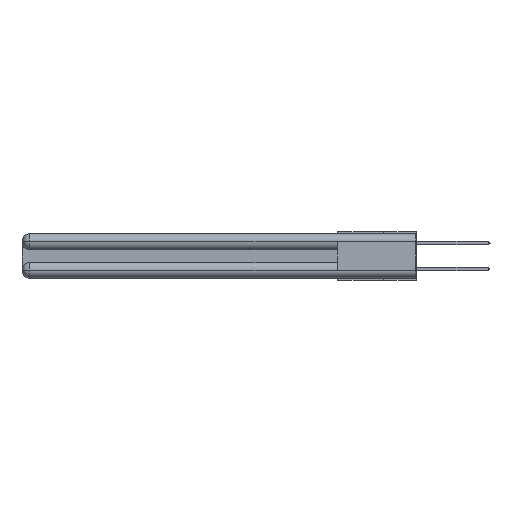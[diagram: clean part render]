
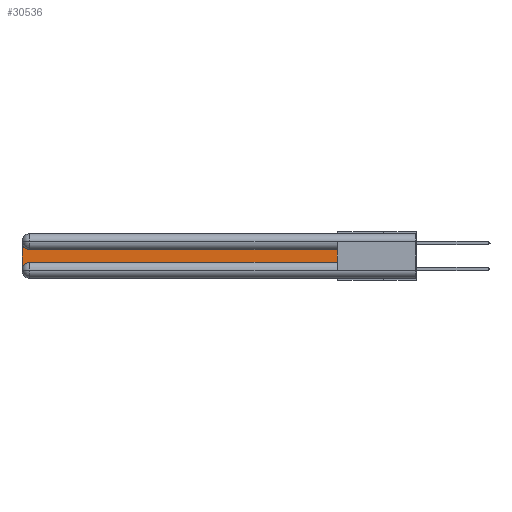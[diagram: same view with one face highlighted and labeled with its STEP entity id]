
A CAD part, left-side view. The second image highlights one B-rep face of the part: STEP entity #30536.
In plain terms, the highlighted planar face has unit normal (-1, 0, 0).
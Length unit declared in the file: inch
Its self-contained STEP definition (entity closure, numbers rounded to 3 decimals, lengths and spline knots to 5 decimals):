
#1309 = LINE ( 'NONE', #4899, #30831 ) ;
#1472 = DIRECTION ( 'NONE',  ( 0., 0., -1. ) ) ;
#1687 = EDGE_CURVE ( 'NONE', #29942, #4841, #17543, .T. ) ;
#2411 = CARTESIAN_POINT ( 'NONE',  ( 0.075, 2.94, -0.2175 ) ) ;
#2611 = CARTESIAN_POINT ( 'NONE',  ( 0.075, 0.6, -0.2175 ) ) ;
#3957 = CIRCLE ( 'NONE', #18396, 0.06 ) ;
#4057 = PLANE ( 'NONE',  #16762 ) ;
#4304 = DIRECTION ( 'NONE',  ( 0., 0., -1. ) ) ;
#4841 = VERTEX_POINT ( 'NONE', #32717 ) ;
#4899 = CARTESIAN_POINT ( 'NONE',  ( 0.075, 3., -0.2175 ) ) ;
#6308 = ORIENTED_EDGE ( 'NONE', *, *, #27136, .T. ) ;
#7314 = DIRECTION ( 'NONE',  ( 0., 0., -1. ) ) ;
#10891 = CARTESIAN_POINT ( 'NONE',  ( 0.075, 0.6, -0.2175 ) ) ;
#12661 = VERTEX_POINT ( 'NONE', #29111 ) ;
#12845 = LINE ( 'NONE', #10891, #14064 ) ;
#13632 = ORIENTED_EDGE ( 'NONE', *, *, #22516, .T. ) ;
#13633 = EDGE_CURVE ( 'NONE', #12661, #31990, #14004, .T. ) ;
#13800 = CARTESIAN_POINT ( 'NONE',  ( 0.075, 2.94, -0.1225 ) ) ;
#13994 = DIRECTION ( 'NONE',  ( 0., 1., 0. ) ) ;
#14004 = LINE ( 'NONE', #2611, #16851 ) ;
#14064 = VECTOR ( 'NONE', #28995, 39.37008 ) ;
#14309 = DIRECTION ( 'NONE',  ( 1., 0., 0. ) ) ;
#14519 = DIRECTION ( 'NONE',  ( 0., 0., -1. ) ) ;
#15681 = ORIENTED_EDGE ( 'NONE', *, *, #16665, .T. ) ;
#16665 = EDGE_CURVE ( 'NONE', #22899, #12661, #12845, .T. ) ;
#16720 = CARTESIAN_POINT ( 'NONE',  ( 0.075, 0.6, -0.1225 ) ) ;
#16762 = AXIS2_PLACEMENT_3D ( 'NONE', #24927, #17221, #14519 ) ;
#16851 = VECTOR ( 'NONE', #28756, 39.37008 ) ;
#17164 = DIRECTION ( 'NONE',  ( 1., 0., 0. ) ) ;
#17221 = DIRECTION ( 'NONE',  ( 1., 0., 0. ) ) ;
#17244 = CARTESIAN_POINT ( 'NONE',  ( 0.075, 2.94, -0.2775 ) ) ;
#17407 = LINE ( 'NONE', #16720, #21937 ) ;
#17543 = CIRCLE ( 'NONE', #22203, 0.06 ) ;
#18396 = AXIS2_PLACEMENT_3D ( 'NONE', #17244, #14309, #4304 ) ;
#19391 = FACE_OUTER_BOUND ( 'NONE', #22889, .T. ) ;
#19636 = ORIENTED_EDGE ( 'NONE', *, *, #13633, .T. ) ;
#21110 = VERTEX_POINT ( 'NONE', #30324 ) ;
#21937 = VECTOR ( 'NONE', #13994, 39.37008 ) ;
#22203 = AXIS2_PLACEMENT_3D ( 'NONE', #32854, #17164, #1472 ) ;
#22516 = EDGE_CURVE ( 'NONE', #21110, #22899, #3957, .T. ) ;
#22889 = EDGE_LOOP ( 'NONE', ( #6308, #23560, #26569, #13632, #15681, #19636 ) ) ;
#22899 = VERTEX_POINT ( 'NONE', #2411 ) ;
#23560 = ORIENTED_EDGE ( 'NONE', *, *, #1687, .T. ) ;
#24927 = CARTESIAN_POINT ( 'NONE',  ( 0.075, 3., -0.1225 ) ) ;
#26447 = CARTESIAN_POINT ( 'NONE',  ( 0.075, 0.6, -0.1225 ) ) ;
#26569 = ORIENTED_EDGE ( 'NONE', *, *, #30413, .T. ) ;
#27136 = EDGE_CURVE ( 'NONE', #31990, #29942, #17407, .T. ) ;
#28756 = DIRECTION ( 'NONE',  ( 0., 0., 1. ) ) ;
#28995 = DIRECTION ( 'NONE',  ( 0., -1., 0. ) ) ;
#29111 = CARTESIAN_POINT ( 'NONE',  ( 0.075, 0.6, -0.2175 ) ) ;
#29942 = VERTEX_POINT ( 'NONE', #13800 ) ;
#30324 = CARTESIAN_POINT ( 'NONE',  ( 0.075, 3., -0.2775 ) ) ;
#30413 = EDGE_CURVE ( 'NONE', #4841, #21110, #1309, .T. ) ;
#30536 = ADVANCED_FACE ( 'NONE', ( #19391 ), #4057, .F. ) ;
#30831 = VECTOR ( 'NONE', #7314, 39.37008 ) ;
#31990 = VERTEX_POINT ( 'NONE', #26447 ) ;
#32717 = CARTESIAN_POINT ( 'NONE',  ( 0.075, 3., -0.0625 ) ) ;
#32854 = CARTESIAN_POINT ( 'NONE',  ( 0.075, 2.94, -0.0625 ) ) ;
